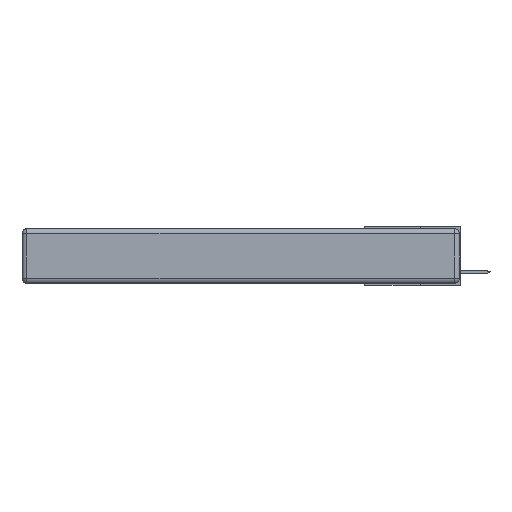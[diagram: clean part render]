
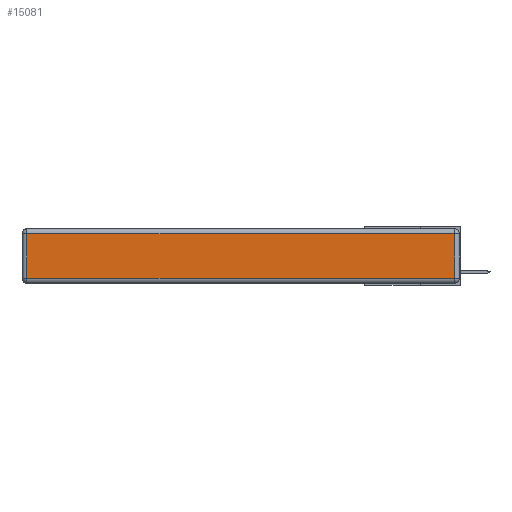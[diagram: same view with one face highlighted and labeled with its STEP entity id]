
A CAD part, left-side view. The second image highlights one B-rep face of the part: STEP entity #15081.
In plain terms, the highlighted planar face has unit normal (-1, 0, 0).
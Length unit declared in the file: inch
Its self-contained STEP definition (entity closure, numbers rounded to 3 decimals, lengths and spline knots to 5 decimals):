
#587 = CARTESIAN_POINT ( 'NONE',  ( 0., 0.03, -0.03 ) ) ;
#895 = VECTOR ( 'NONE', #30168, 39.37008 ) ;
#3127 = EDGE_LOOP ( 'NONE', ( #30607, #31819, #30034, #22090 ) ) ;
#3639 = DIRECTION ( 'NONE',  ( 0., 0., 1. ) ) ;
#4358 = CARTESIAN_POINT ( 'NONE',  ( 0., 0.03, -0.343 ) ) ;
#4464 = DIRECTION ( 'NONE',  ( 0., 0., 1. ) ) ;
#5175 = DIRECTION ( 'NONE',  ( 0., 0., -1. ) ) ;
#5871 = VECTOR ( 'NONE', #5175, 39.37008 ) ;
#7166 = CARTESIAN_POINT ( 'NONE',  ( 0., 2.72, -0.03 ) ) ;
#7818 = CARTESIAN_POINT ( 'NONE',  ( 0., 2.72, -0.343 ) ) ;
#9282 = EDGE_CURVE ( 'NONE', #11798, #15567, #29828, .T. ) ;
#11798 = VERTEX_POINT ( 'NONE', #587 ) ;
#12160 = LINE ( 'NONE', #7818, #5871 ) ;
#13238 = DIRECTION ( 'NONE',  ( -1., 0., 0. ) ) ;
#14797 = VECTOR ( 'NONE', #4464, 39.37008 ) ;
#14839 = VERTEX_POINT ( 'NONE', #31623 ) ;
#15081 = ADVANCED_FACE ( 'NONE', ( #23499 ), #23469, .T. ) ;
#15567 = VERTEX_POINT ( 'NONE', #7166 ) ;
#15605 = LINE ( 'NONE', #4358, #14797 ) ;
#15855 = AXIS2_PLACEMENT_3D ( 'NONE', #28806, #13238, #3639 ) ;
#17114 = EDGE_CURVE ( 'NONE', #15567, #14839, #12160, .T. ) ;
#18968 = CARTESIAN_POINT ( 'NONE',  ( 0., 0.03, -0.313 ) ) ;
#19924 = LINE ( 'NONE', #27307, #25059 ) ;
#20561 = EDGE_CURVE ( 'NONE', #14839, #26935, #19924, .T. ) ;
#21721 = EDGE_CURVE ( 'NONE', #26935, #11798, #15605, .T. ) ;
#22090 = ORIENTED_EDGE ( 'NONE', *, *, #17114, .T. ) ;
#23469 = PLANE ( 'NONE',  #15855 ) ;
#23499 = FACE_OUTER_BOUND ( 'NONE', #3127, .T. ) ;
#24630 = DIRECTION ( 'NONE',  ( 0., -1., 0. ) ) ;
#25059 = VECTOR ( 'NONE', #24630, 39.37008 ) ;
#26935 = VERTEX_POINT ( 'NONE', #18968 ) ;
#27307 = CARTESIAN_POINT ( 'NONE',  ( 0., 0., -0.313 ) ) ;
#27378 = CARTESIAN_POINT ( 'NONE',  ( 0., 2.75, -0.03 ) ) ;
#28806 = CARTESIAN_POINT ( 'NONE',  ( 0., 0., -0.343 ) ) ;
#29828 = LINE ( 'NONE', #27378, #895 ) ;
#30034 = ORIENTED_EDGE ( 'NONE', *, *, #9282, .T. ) ;
#30168 = DIRECTION ( 'NONE',  ( 0., 1., 0. ) ) ;
#30607 = ORIENTED_EDGE ( 'NONE', *, *, #20561, .T. ) ;
#31623 = CARTESIAN_POINT ( 'NONE',  ( 0., 2.72, -0.313 ) ) ;
#31819 = ORIENTED_EDGE ( 'NONE', *, *, #21721, .T. ) ;
